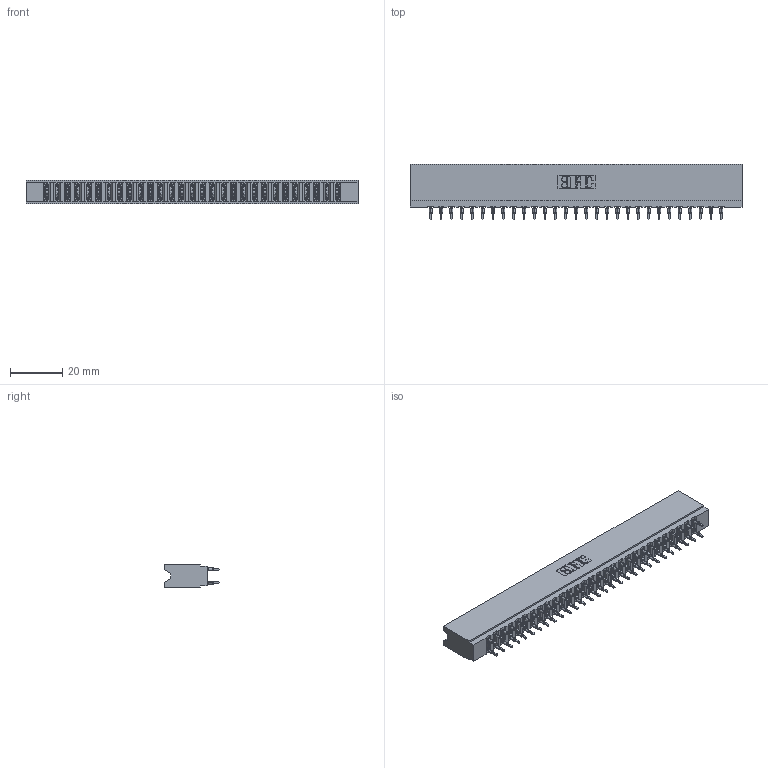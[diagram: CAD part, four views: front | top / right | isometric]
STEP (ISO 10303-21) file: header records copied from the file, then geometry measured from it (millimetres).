
FILE_DESCRIPTION (( 'STEP AP203' ), '1' );
FILE_NAME ('737-058-560-206.STEP', '2020-09-11T05:39:19', ( '' ), ( '' ), 'SwSTEP 2.0', 'SolidWorks 2020', '' );
FILE_SCHEMA (( 'CONFIG_CONTROL_DESIGN' ));
Length unit declared in the file: inch
Products named in the file (3): 737-058-560-206; 745-292-001_560; 737 Part_Insulator Option - 06
Assembly tree (59 placements, depth 2):
  737-058-560-206
    737 Part_Insulator Option - 06
    745-292-001_560  x58
Bounding box: 126.75 x 21.22 x 8.89 mm (x, y, z)
Volume: 12804.4 mm3; surface area: 19361 mm2
Topology: 59 solids, 59 shells, 5837 faces, 15975 edges, 10146 vertices
Faces by surface type: plane 3042, cylinder 1287, bspline 1160, torus 348
Entity records: 51870 total; most frequent: CARTESIAN_POINT 9512, ORIENTED_EDGE 8922, DIRECTION 7803, EDGE_CURVE 4461, VECTOR 4097, LINE 4097, VERTEX_POINT 2850, AXIS2_PLACEMENT_3D 1853
